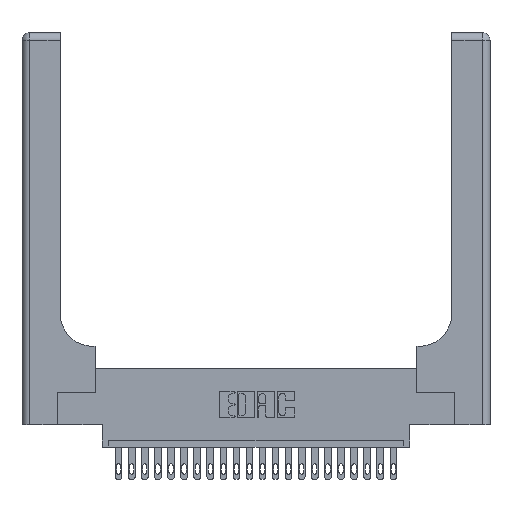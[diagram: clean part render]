
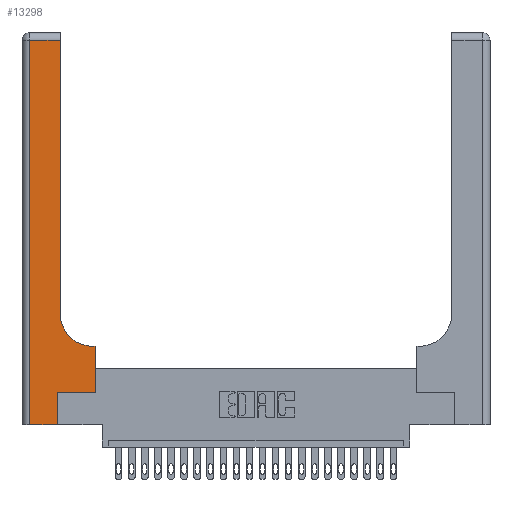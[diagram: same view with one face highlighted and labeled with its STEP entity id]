
A CAD part, top view. The second image highlights one B-rep face of the part: STEP entity #13298.
In plain terms, the highlighted planar face has unit normal (0, 0, 1).
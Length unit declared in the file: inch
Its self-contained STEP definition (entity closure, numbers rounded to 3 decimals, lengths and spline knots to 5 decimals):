
#713 = CARTESIAN_POINT ( 'NONE',  ( 0.269, 0.25, 0.37 ) ) ;
#1000 = CARTESIAN_POINT ( 'NONE',  ( 0.269, 0., 0.37 ) ) ;
#1015 = CARTESIAN_POINT ( 'NONE',  ( 0.5585, 0.25, 0.37 ) ) ;
#1675 = ORIENTED_EDGE ( 'NONE', *, *, #20111, .T. ) ;
#2013 = VECTOR ( 'NONE', #5210, 39.37008 ) ;
#2648 = DIRECTION ( 'NONE',  ( 0., 1., 0. ) ) ;
#3089 = VECTOR ( 'NONE', #18273, 39.37008 ) ;
#3195 = LINE ( 'NONE', #1015, #6744 ) ;
#3348 = ORIENTED_EDGE ( 'NONE', *, *, #11012, .T. ) ;
#4414 = VECTOR ( 'NONE', #19005, 39.37008 ) ;
#4626 = CARTESIAN_POINT ( 'NONE',  ( 0.06, 2.94, 0.37 ) ) ;
#4670 = ORIENTED_EDGE ( 'NONE', *, *, #11779, .T. ) ;
#5170 = AXIS2_PLACEMENT_3D ( 'NONE', #19445, #23485, #10004 ) ;
#5210 = DIRECTION ( 'NONE',  ( 0., 1., 0. ) ) ;
#6341 = VERTEX_POINT ( 'NONE', #10640 ) ;
#6743 = EDGE_CURVE ( 'NONE', #9061, #20127, #15353, .T. ) ;
#6744 = VECTOR ( 'NONE', #12247, 39.37008 ) ;
#7013 = CARTESIAN_POINT ( 'NONE',  ( 0.5585, 0.6, 0.37 ) ) ;
#7291 = CARTESIAN_POINT ( 'NONE',  ( 0.06, 0., 0.37 ) ) ;
#7358 = LINE ( 'NONE', #7738, #16220 ) ;
#7489 = EDGE_CURVE ( 'NONE', #8453, #18903, #7358, .T. ) ;
#7677 = EDGE_CURVE ( 'NONE', #17648, #8453, #11741, .T. ) ;
#7738 = CARTESIAN_POINT ( 'NONE',  ( 0.06, 3., 0.37 ) ) ;
#8453 = VERTEX_POINT ( 'NONE', #4626 ) ;
#8505 = DIRECTION ( 'NONE',  ( -1., 0., 0. ) ) ;
#8662 = VECTOR ( 'NONE', #15467, 39.37008 ) ;
#9061 = VERTEX_POINT ( 'NONE', #713 ) ;
#9222 = LINE ( 'NONE', #17900, #8662 ) ;
#9478 = ORIENTED_EDGE ( 'NONE', *, *, #20015, .T. ) ;
#10004 = DIRECTION ( 'NONE',  ( 1., 0., 0. ) ) ;
#10640 = CARTESIAN_POINT ( 'NONE',  ( 0.2915, 0.85, 0.37 ) ) ;
#10696 = CIRCLE ( 'NONE', #5170, 0.25 ) ;
#11012 = EDGE_CURVE ( 'NONE', #18903, #16664, #9222, .T. ) ;
#11287 = DIRECTION ( 'NONE',  ( 0., -1., 0. ) ) ;
#11380 = ORIENTED_EDGE ( 'NONE', *, *, #18746, .T. ) ;
#11632 = ORIENTED_EDGE ( 'NONE', *, *, #7677, .T. ) ;
#11741 = LINE ( 'NONE', #24385, #12921 ) ;
#11779 = EDGE_CURVE ( 'NONE', #15774, #6341, #10696, .T. ) ;
#12247 = DIRECTION ( 'NONE',  ( 0., 1., 0. ) ) ;
#12866 = CARTESIAN_POINT ( 'NONE',  ( 0.5415, 0.6, 0.37 ) ) ;
#12885 = CARTESIAN_POINT ( 'NONE',  ( 0.5585, 0.25, 0.37 ) ) ;
#12921 = VECTOR ( 'NONE', #8505, 39.37008 ) ;
#13298 = ADVANCED_FACE ( 'NONE', ( #14554 ), #18085, .F. ) ;
#14208 = DIRECTION ( 'NONE',  ( 0., 0., -1. ) ) ;
#14554 = FACE_OUTER_BOUND ( 'NONE', #16417, .T. ) ;
#14611 = ORIENTED_EDGE ( 'NONE', *, *, #7489, .T. ) ;
#14714 = LINE ( 'NONE', #21784, #2013 ) ;
#15144 = EDGE_CURVE ( 'NONE', #6341, #17648, #23639, .T. ) ;
#15155 = AXIS2_PLACEMENT_3D ( 'NONE', #23778, #14208, #19735 ) ;
#15353 = LINE ( 'NONE', #20935, #4414 ) ;
#15467 = DIRECTION ( 'NONE',  ( 1., 0., 0. ) ) ;
#15774 = VERTEX_POINT ( 'NONE', #12866 ) ;
#16220 = VECTOR ( 'NONE', #11287, 39.37008 ) ;
#16417 = EDGE_LOOP ( 'NONE', ( #22251, #11632, #14611, #3348, #1675, #20091, #9478, #11380, #4670 ) ) ;
#16664 = VERTEX_POINT ( 'NONE', #1000 ) ;
#17648 = VERTEX_POINT ( 'NONE', #18473 ) ;
#17900 = CARTESIAN_POINT ( 'NONE',  ( 0., 0., 0.37 ) ) ;
#18085 = PLANE ( 'NONE',  #15155 ) ;
#18273 = DIRECTION ( 'NONE',  ( -1., 0., 0. ) ) ;
#18473 = CARTESIAN_POINT ( 'NONE',  ( 0.2915, 2.94, 0.37 ) ) ;
#18746 = EDGE_CURVE ( 'NONE', #21975, #15774, #20546, .T. ) ;
#18903 = VERTEX_POINT ( 'NONE', #7291 ) ;
#19005 = DIRECTION ( 'NONE',  ( 1., 0., 0. ) ) ;
#19445 = CARTESIAN_POINT ( 'NONE',  ( 0.5415, 0.85, 0.37 ) ) ;
#19735 = DIRECTION ( 'NONE',  ( -1., 0., 0. ) ) ;
#20015 = EDGE_CURVE ( 'NONE', #20127, #21975, #3195, .T. ) ;
#20091 = ORIENTED_EDGE ( 'NONE', *, *, #6743, .T. ) ;
#20111 = EDGE_CURVE ( 'NONE', #16664, #9061, #14714, .T. ) ;
#20127 = VERTEX_POINT ( 'NONE', #12885 ) ;
#20333 = CARTESIAN_POINT ( 'NONE',  ( 0.2915, 0.6, 0.37 ) ) ;
#20546 = LINE ( 'NONE', #20333, #3089 ) ;
#20935 = CARTESIAN_POINT ( 'NONE',  ( 0.269, 0.25, 0.37 ) ) ;
#21270 = CARTESIAN_POINT ( 'NONE',  ( 0.2915, 3., 0.37 ) ) ;
#21784 = CARTESIAN_POINT ( 'NONE',  ( 0.269, 0., 0.37 ) ) ;
#21975 = VERTEX_POINT ( 'NONE', #7013 ) ;
#22251 = ORIENTED_EDGE ( 'NONE', *, *, #15144, .T. ) ;
#22435 = VECTOR ( 'NONE', #2648, 39.37008 ) ;
#23485 = DIRECTION ( 'NONE',  ( 0., 0., -1. ) ) ;
#23639 = LINE ( 'NONE', #21270, #22435 ) ;
#23778 = CARTESIAN_POINT ( 'NONE',  ( 0., 3., 0.37 ) ) ;
#24385 = CARTESIAN_POINT ( 'NONE',  ( 0., 2.94, 0.37 ) ) ;
